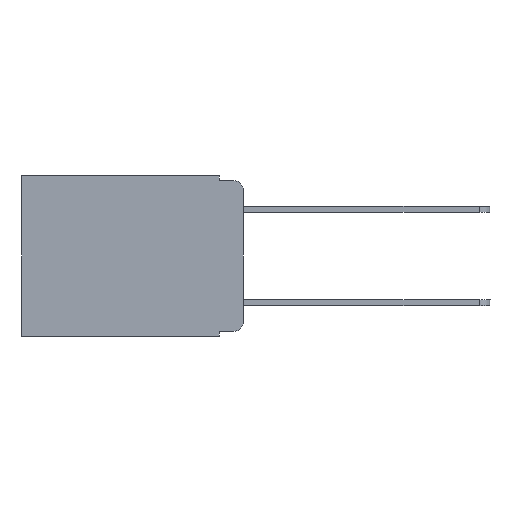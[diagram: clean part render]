
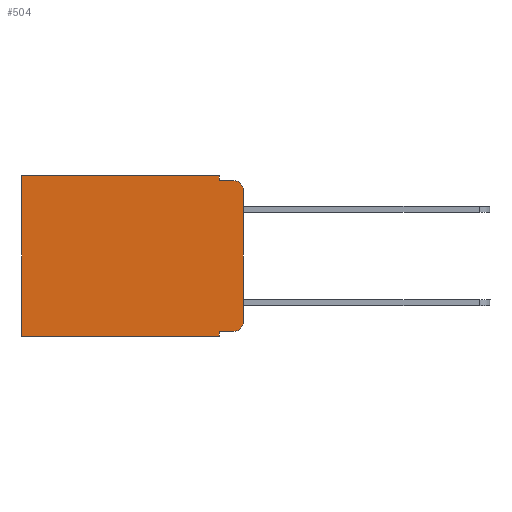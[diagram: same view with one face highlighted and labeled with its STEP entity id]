
A CAD part, left-side view. The second image highlights one B-rep face of the part: STEP entity #504.
In plain terms, the highlighted planar face has unit normal (-1, 0, 0).
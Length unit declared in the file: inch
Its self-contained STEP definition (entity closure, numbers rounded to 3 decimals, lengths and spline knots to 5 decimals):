
#29 = VERTEX_POINT ( 'NONE', #9703 ) ;
#31 = CARTESIAN_POINT ( 'NONE',  ( 0.298, 0., 0. ) ) ;
#172 = CARTESIAN_POINT ( 'NONE',  ( 0.298, 0.02, -0.313 ) ) ;
#194 = CARTESIAN_POINT ( 'NONE',  ( 0.298, 0.02, -0.03 ) ) ;
#291 = LINE ( 'NONE', #6713, #8570 ) ;
#301 = PLANE ( 'NONE',  #8949 ) ;
#316 = VECTOR ( 'NONE', #9970, 39.37008 ) ;
#504 = ADVANCED_FACE ( 'NONE', ( #1138 ), #301, .F. ) ;
#583 = DIRECTION ( 'NONE',  ( 0., 0., -1. ) ) ;
#846 = ORIENTED_EDGE ( 'NONE', *, *, #7250, .F. ) ;
#953 = LINE ( 'NONE', #5717, #1052 ) ;
#975 = DIRECTION ( 'NONE',  ( 0., 0., -1. ) ) ;
#1052 = VECTOR ( 'NONE', #8920, 39.37008 ) ;
#1093 = VERTEX_POINT ( 'NONE', #1341 ) ;
#1138 = FACE_OUTER_BOUND ( 'NONE', #5524, .T. ) ;
#1171 = VERTEX_POINT ( 'NONE', #2434 ) ;
#1292 = ORIENTED_EDGE ( 'NONE', *, *, #5116, .T. ) ;
#1341 = CARTESIAN_POINT ( 'NONE',  ( 0.298, 0.473, -0.343 ) ) ;
#1981 = DIRECTION ( 'NONE',  ( 0., -1., 0. ) ) ;
#2141 = LINE ( 'NONE', #9981, #4529 ) ;
#2149 = CIRCLE ( 'NONE', #7940, 0.02 ) ;
#2413 = VERTEX_POINT ( 'NONE', #2592 ) ;
#2434 = CARTESIAN_POINT ( 'NONE',  ( 0.298, 0.02, -0.333 ) ) ;
#2449 = LINE ( 'NONE', #31, #7906 ) ;
#2544 = ORIENTED_EDGE ( 'NONE', *, *, #7644, .F. ) ;
#2592 = CARTESIAN_POINT ( 'NONE',  ( 0.298, 0.02, -0.01 ) ) ;
#2945 = DIRECTION ( 'NONE',  ( 0., 0., -1. ) ) ;
#3096 = VECTOR ( 'NONE', #4196, 39.37008 ) ;
#3413 = VECTOR ( 'NONE', #583, 39.37008 ) ;
#3517 = EDGE_CURVE ( 'NONE', #7758, #29, #953, .T. ) ;
#3547 = VERTEX_POINT ( 'NONE', #8395 ) ;
#3600 = CARTESIAN_POINT ( 'NONE',  ( 0.298, 0., -0.343 ) ) ;
#3919 = CARTESIAN_POINT ( 'NONE',  ( 0.298, 0.051, -0.01 ) ) ;
#3978 = DIRECTION ( 'NONE',  ( -1., 0., 0. ) ) ;
#4061 = VECTOR ( 'NONE', #2945, 39.37008 ) ;
#4196 = DIRECTION ( 'NONE',  ( 0., -1., 0. ) ) ;
#4365 = DIRECTION ( 'NONE',  ( 1., 0., 0. ) ) ;
#4450 = LINE ( 'NONE', #8400, #4061 ) ;
#4506 = CARTESIAN_POINT ( 'NONE',  ( 0.298, 0.473, 0. ) ) ;
#4529 = VECTOR ( 'NONE', #6080, 39.37008 ) ;
#4658 = EDGE_CURVE ( 'NONE', #3547, #6454, #2449, .T. ) ;
#4775 = EDGE_CURVE ( 'NONE', #6454, #1093, #5297, .T. ) ;
#4801 = DIRECTION ( 'NONE',  ( 0., 0., -1. ) ) ;
#5021 = EDGE_CURVE ( 'NONE', #7758, #2413, #7575, .T. ) ;
#5046 = EDGE_CURVE ( 'NONE', #7374, #2413, #9624, .T. ) ;
#5116 = EDGE_CURVE ( 'NONE', #6102, #1171, #291, .T. ) ;
#5238 = ORIENTED_EDGE ( 'NONE', *, *, #4658, .T. ) ;
#5297 = LINE ( 'NONE', #10058, #3413 ) ;
#5524 = EDGE_LOOP ( 'NONE', ( #9393, #9722, #8675, #2544, #5238, #7781, #8466, #846, #1292, #8849 ) ) ;
#5620 = CARTESIAN_POINT ( 'NONE',  ( 0.298, 0.051, -0.333 ) ) ;
#5717 = CARTESIAN_POINT ( 'NONE',  ( 0.298, 0., 0. ) ) ;
#5938 = CARTESIAN_POINT ( 'NONE',  ( 0.298, 0., 0. ) ) ;
#6080 = DIRECTION ( 'NONE',  ( 0., 0., -1. ) ) ;
#6102 = VERTEX_POINT ( 'NONE', #5620 ) ;
#6165 = VERTEX_POINT ( 'NONE', #8714 ) ;
#6380 = EDGE_CURVE ( 'NONE', #6165, #1093, #6904, .T. ) ;
#6454 = VERTEX_POINT ( 'NONE', #4506 ) ;
#6713 = CARTESIAN_POINT ( 'NONE',  ( 0.298, 0.051, -0.333 ) ) ;
#6904 = LINE ( 'NONE', #3600, #316 ) ;
#7062 = DIRECTION ( 'NONE',  ( -1., 0., 0. ) ) ;
#7226 = CARTESIAN_POINT ( 'NONE',  ( 0.298, 0., -0.03 ) ) ;
#7250 = EDGE_CURVE ( 'NONE', #6102, #6165, #2141, .T. ) ;
#7374 = VERTEX_POINT ( 'NONE', #3919 ) ;
#7575 = CIRCLE ( 'NONE', #10023, 0.02 ) ;
#7644 = EDGE_CURVE ( 'NONE', #3547, #7374, #4450, .T. ) ;
#7758 = VERTEX_POINT ( 'NONE', #7226 ) ;
#7781 = ORIENTED_EDGE ( 'NONE', *, *, #4775, .T. ) ;
#7856 = EDGE_CURVE ( 'NONE', #1171, #29, #2149, .T. ) ;
#7906 = VECTOR ( 'NONE', #9522, 39.37008 ) ;
#7940 = AXIS2_PLACEMENT_3D ( 'NONE', #172, #7062, #4801 ) ;
#8395 = CARTESIAN_POINT ( 'NONE',  ( 0.298, 0.051, 0. ) ) ;
#8400 = CARTESIAN_POINT ( 'NONE',  ( 0.298, 0.051, 0. ) ) ;
#8466 = ORIENTED_EDGE ( 'NONE', *, *, #6380, .F. ) ;
#8570 = VECTOR ( 'NONE', #1981, 39.37008 ) ;
#8675 = ORIENTED_EDGE ( 'NONE', *, *, #5046, .F. ) ;
#8714 = CARTESIAN_POINT ( 'NONE',  ( 0.298, 0.051, -0.343 ) ) ;
#8828 = DIRECTION ( 'NONE',  ( 0., 0., -1. ) ) ;
#8849 = ORIENTED_EDGE ( 'NONE', *, *, #7856, .T. ) ;
#8873 = CARTESIAN_POINT ( 'NONE',  ( 0.298, 0.051, -0.01 ) ) ;
#8920 = DIRECTION ( 'NONE',  ( 0., 0., -1. ) ) ;
#8949 = AXIS2_PLACEMENT_3D ( 'NONE', #5938, #4365, #975 ) ;
#9393 = ORIENTED_EDGE ( 'NONE', *, *, #3517, .F. ) ;
#9522 = DIRECTION ( 'NONE',  ( 0., 1., 0. ) ) ;
#9624 = LINE ( 'NONE', #8873, #3096 ) ;
#9703 = CARTESIAN_POINT ( 'NONE',  ( 0.298, 0., -0.313 ) ) ;
#9722 = ORIENTED_EDGE ( 'NONE', *, *, #5021, .T. ) ;
#9970 = DIRECTION ( 'NONE',  ( 0., 1., 0. ) ) ;
#9981 = CARTESIAN_POINT ( 'NONE',  ( 0.298, 0.051, 0. ) ) ;
#10023 = AXIS2_PLACEMENT_3D ( 'NONE', #194, #3978, #8828 ) ;
#10058 = CARTESIAN_POINT ( 'NONE',  ( 0.298, 0.473, 0. ) ) ;
